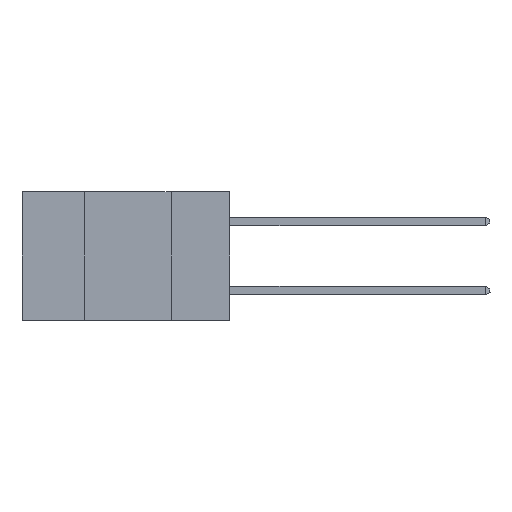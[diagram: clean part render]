
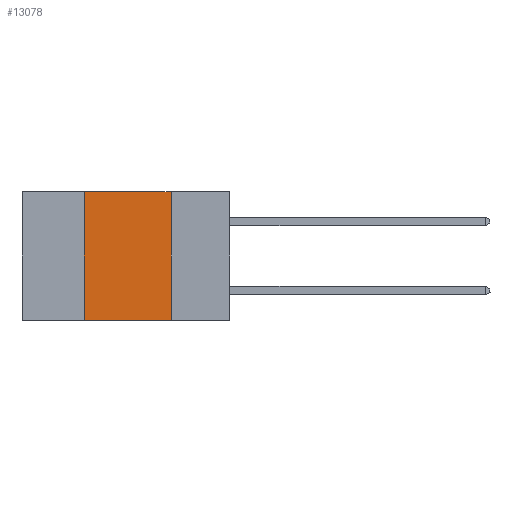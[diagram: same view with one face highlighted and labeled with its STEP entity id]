
A CAD part, left-side view. The second image highlights one B-rep face of the part: STEP entity #13078.
In plain terms, the highlighted planar face has unit normal (-1, 0, 0).
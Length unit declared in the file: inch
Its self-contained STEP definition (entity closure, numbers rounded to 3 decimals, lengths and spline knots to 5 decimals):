
#1180 = VECTOR ( 'NONE', #22708, 39.37008 ) ;
#1223 = CARTESIAN_POINT ( 'NONE',  ( 0., 0.42, -0.37 ) ) ;
#4057 = EDGE_CURVE ( 'NONE', #7260, #13745, #14286, .T. ) ;
#4657 = VERTEX_POINT ( 'NONE', #16927 ) ;
#5316 = VECTOR ( 'NONE', #18616, 39.37008 ) ;
#5621 = DIRECTION ( 'NONE',  ( 1., 0., 0. ) ) ;
#5870 = EDGE_CURVE ( 'NONE', #7260, #9081, #13080, .T. ) ;
#6502 = LINE ( 'NONE', #12737, #5316 ) ;
#7260 = VERTEX_POINT ( 'NONE', #1223 ) ;
#7515 = CARTESIAN_POINT ( 'NONE',  ( 0., 0.42, 0. ) ) ;
#8026 = VECTOR ( 'NONE', #10370, 39.37008 ) ;
#9081 = VERTEX_POINT ( 'NONE', #22148 ) ;
#9958 = LINE ( 'NONE', #11728, #18924 ) ;
#10370 = DIRECTION ( 'NONE',  ( 0., -1., 0. ) ) ;
#11468 = PLANE ( 'NONE',  #16878 ) ;
#11728 = CARTESIAN_POINT ( 'NONE',  ( 0., 0.17, 0. ) ) ;
#12737 = CARTESIAN_POINT ( 'NONE',  ( 0., 0.6, 0. ) ) ;
#12751 = ORIENTED_EDGE ( 'NONE', *, *, #19754, .F. ) ;
#13078 = ADVANCED_FACE ( 'NONE', ( #14666 ), #11468, .F. ) ;
#13080 = LINE ( 'NONE', #17400, #8026 ) ;
#13291 = CARTESIAN_POINT ( 'NONE',  ( 0., 0.42, 0. ) ) ;
#13411 = EDGE_LOOP ( 'NONE', ( #12751, #15311, #13808, #22728 ) ) ;
#13745 = VERTEX_POINT ( 'NONE', #13291 ) ;
#13808 = ORIENTED_EDGE ( 'NONE', *, *, #4057, .F. ) ;
#14286 = LINE ( 'NONE', #7515, #1180 ) ;
#14666 = FACE_OUTER_BOUND ( 'NONE', #13411, .T. ) ;
#15311 = ORIENTED_EDGE ( 'NONE', *, *, #16495, .F. ) ;
#16495 = EDGE_CURVE ( 'NONE', #13745, #4657, #6502, .T. ) ;
#16878 = AXIS2_PLACEMENT_3D ( 'NONE', #22836, #5621, #21000 ) ;
#16927 = CARTESIAN_POINT ( 'NONE',  ( 0., 0.17, 0. ) ) ;
#17400 = CARTESIAN_POINT ( 'NONE',  ( 0., 0.6, -0.37 ) ) ;
#17658 = DIRECTION ( 'NONE',  ( 0., 0., -1. ) ) ;
#18616 = DIRECTION ( 'NONE',  ( 0., -1., 0. ) ) ;
#18924 = VECTOR ( 'NONE', #17658, 39.37008 ) ;
#19754 = EDGE_CURVE ( 'NONE', #4657, #9081, #9958, .T. ) ;
#21000 = DIRECTION ( 'NONE',  ( 0., 0., -1. ) ) ;
#22148 = CARTESIAN_POINT ( 'NONE',  ( 0., 0.17, -0.37 ) ) ;
#22708 = DIRECTION ( 'NONE',  ( 0., 0., 1. ) ) ;
#22728 = ORIENTED_EDGE ( 'NONE', *, *, #5870, .T. ) ;
#22836 = CARTESIAN_POINT ( 'NONE',  ( 0., 0.6, 0. ) ) ;
